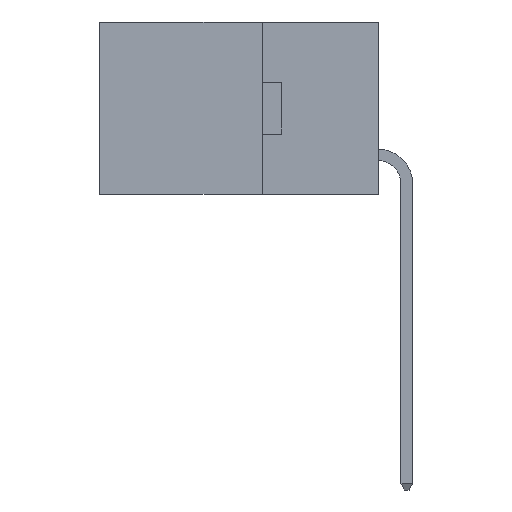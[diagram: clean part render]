
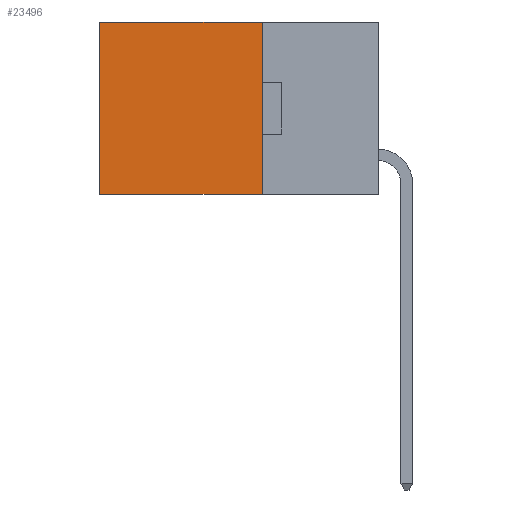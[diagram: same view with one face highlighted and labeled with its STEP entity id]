
A CAD part, left-side view. The second image highlights one B-rep face of the part: STEP entity #23496.
In plain terms, the highlighted planar face has unit normal (-1, 0, 0).
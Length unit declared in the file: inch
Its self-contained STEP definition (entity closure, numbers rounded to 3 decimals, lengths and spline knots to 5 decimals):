
#706 = EDGE_CURVE ( 'NONE', #23320, #19751, #20713, .T. ) ;
#874 = EDGE_CURVE ( 'NONE', #19638, #23320, #22295, .T. ) ;
#1358 = CARTESIAN_POINT ( 'NONE',  ( 0.2615, 0.25, -0.37 ) ) ;
#2342 = CARTESIAN_POINT ( 'NONE',  ( 0.2615, 0.6, -0.37 ) ) ;
#2513 = VECTOR ( 'NONE', #21733, 39.37008 ) ;
#3213 = EDGE_LOOP ( 'NONE', ( #8208, #10266, #15517, #8158 ) ) ;
#3821 = PLANE ( 'NONE',  #6710 ) ;
#4683 = VECTOR ( 'NONE', #5617, 39.37008 ) ;
#5617 = DIRECTION ( 'NONE',  ( 0., 0., -1. ) ) ;
#5924 = DIRECTION ( 'NONE',  ( 1., 0., 0. ) ) ;
#6172 = CARTESIAN_POINT ( 'NONE',  ( 0.2615, 0.25, -0.37 ) ) ;
#6710 = AXIS2_PLACEMENT_3D ( 'NONE', #26093, #5924, #20054 ) ;
#8158 = ORIENTED_EDGE ( 'NONE', *, *, #874, .T. ) ;
#8208 = ORIENTED_EDGE ( 'NONE', *, *, #706, .T. ) ;
#9999 = DIRECTION ( 'NONE',  ( 0., 1., 0. ) ) ;
#10266 = ORIENTED_EDGE ( 'NONE', *, *, #22135, .F. ) ;
#11040 = VECTOR ( 'NONE', #9999, 39.37008 ) ;
#11133 = CARTESIAN_POINT ( 'NONE',  ( 0.2615, 0.6, -0.37 ) ) ;
#12088 = CARTESIAN_POINT ( 'NONE',  ( 0.2615, 0.25, 0. ) ) ;
#13728 = CARTESIAN_POINT ( 'NONE',  ( 0.2615, 0.25, -0.37 ) ) ;
#14277 = CARTESIAN_POINT ( 'NONE',  ( 0.2615, 0.25, 0. ) ) ;
#15517 = ORIENTED_EDGE ( 'NONE', *, *, #16051, .F. ) ;
#16040 = VECTOR ( 'NONE', #17191, 39.37008 ) ;
#16051 = EDGE_CURVE ( 'NONE', #19638, #20322, #20852, .T. ) ;
#17191 = DIRECTION ( 'NONE',  ( 0., 0., -1. ) ) ;
#18324 = FACE_OUTER_BOUND ( 'NONE', #3213, .T. ) ;
#19387 = LINE ( 'NONE', #13728, #2513 ) ;
#19443 = CARTESIAN_POINT ( 'NONE',  ( 0.2615, 0.6, 0. ) ) ;
#19638 = VERTEX_POINT ( 'NONE', #14277 ) ;
#19751 = VERTEX_POINT ( 'NONE', #2342 ) ;
#20054 = DIRECTION ( 'NONE',  ( 0., 0., -1. ) ) ;
#20322 = VERTEX_POINT ( 'NONE', #6172 ) ;
#20713 = LINE ( 'NONE', #11133, #16040 ) ;
#20852 = LINE ( 'NONE', #1358, #4683 ) ;
#21733 = DIRECTION ( 'NONE',  ( 0., 1., 0. ) ) ;
#22135 = EDGE_CURVE ( 'NONE', #20322, #19751, #19387, .T. ) ;
#22295 = LINE ( 'NONE', #12088, #11040 ) ;
#23320 = VERTEX_POINT ( 'NONE', #19443 ) ;
#23496 = ADVANCED_FACE ( 'NONE', ( #18324 ), #3821, .F. ) ;
#26093 = CARTESIAN_POINT ( 'NONE',  ( 0.2615, 0.25, -0.37 ) ) ;
